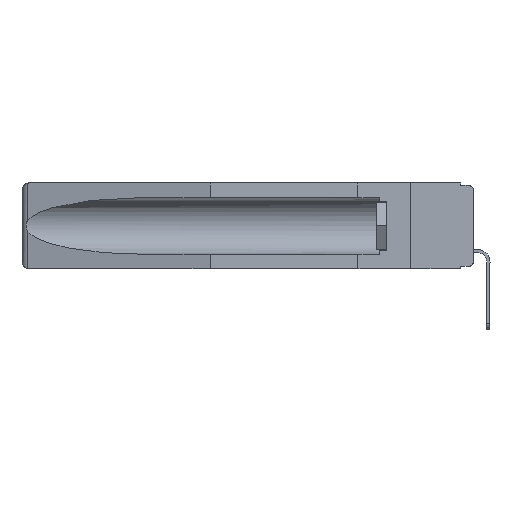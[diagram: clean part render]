
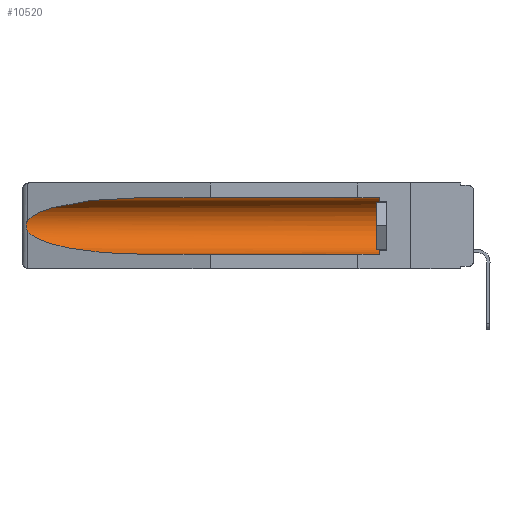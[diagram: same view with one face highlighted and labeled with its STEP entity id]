
A CAD part, left-side view. The second image highlights one B-rep face of the part: STEP entity #10520.
In plain terms, the highlighted cylindrical face has radius 2.857 mm (diameter 5.715 mm), a partial arc.
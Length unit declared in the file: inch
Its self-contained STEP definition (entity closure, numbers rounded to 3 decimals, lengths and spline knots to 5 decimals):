
#269 = VERTEX_POINT ( 'NONE', #14344 ) ;
#303 = DIRECTION ( 'NONE',  ( 0., 1., 0. ) ) ;
#357 = CYLINDRICAL_SURFACE ( 'NONE', #995, 0.1125 ) ;
#407 = CARTESIAN_POINT ( 'NONE',  ( 0.2675, 1.53308, -0.16763 ) ) ;
#995 = AXIS2_PLACEMENT_3D ( 'NONE', #14981, #9896, #12341 ) ;
#1066 = VECTOR ( 'NONE', #303, 39.37008 ) ;
#1364 = VERTEX_POINT ( 'NONE', #14664 ) ;
#1693 = EDGE_CURVE ( 'NONE', #8543, #269, #13814, .T. ) ;
#2449 = EDGE_CURVE ( 'NONE', #1364, #11812, #15150, .T. ) ;
#2573 = CARTESIAN_POINT ( 'NONE',  ( 0.155, 0.126, -0.1715 ) ) ;
#2664 = VERTEX_POINT ( 'NONE', #16634 ) ;
#2961 = CARTESIAN_POINT ( 'NONE',  ( 0.26537, 1.52718, -0.19328 ) ) ;
#3813 = CARTESIAN_POINT ( 'NONE',  ( 0.25451, 1.48313, -0.24835 ) ) ;
#4044 = ORIENTED_EDGE ( 'NONE', *, *, #7156, .T. ) ;
#4131 = ORIENTED_EDGE ( 'NONE', *, *, #1693, .T. ) ;
#4334 = CARTESIAN_POINT ( 'NONE',  ( 0.155, -0.30754, -0.284 ) ) ;
#4537 = CARTESIAN_POINT ( 'NONE',  ( 0.26597, 1.5296, -0.19026 ) ) ;
#4925 = CARTESIAN_POINT ( 'NONE',  ( 0.155, 1.07973, -0.059 ) ) ;
#6120 = CARTESIAN_POINT ( 'NONE',  ( 0.155, -0.30754, -0.059 ) ) ;
#6208 = ORIENTED_EDGE ( 'NONE', *, *, #2449, .T. ) ;
#6341 = CARTESIAN_POINT ( 'NONE',  ( 0.25451, 1.48313, -0.09465 ) ) ;
#6611 = DIRECTION ( 'NONE',  ( 0., -1., 0. ) ) ;
#7156 = EDGE_CURVE ( 'NONE', #2664, #10447, #7254, .T. ) ;
#7173 = CARTESIAN_POINT ( 'NONE',  ( 0.26597, 1.52961, -0.15275 ) ) ;
#7254 =( BOUNDED_CURVE ( )  B_SPLINE_CURVE ( 3, ( #10452, #3813, #14580, #13158 ),
 .UNSPECIFIED., .F., .F. ) 
 B_SPLINE_CURVE_WITH_KNOTS ( ( 4, 4 ),
 ( 0.1948, 1.5708 ),
 .UNSPECIFIED. ) 
 CURVE ( )  GEOMETRIC_REPRESENTATION_ITEM ( )  RATIONAL_B_SPLINE_CURVE ( ( 1., 0.848, 0.848, 1. ) ) 
 REPRESENTATION_ITEM ( '' )  );
#7483 = CARTESIAN_POINT ( 'NONE',  ( 0.26654, 1.53092, -0.15636 ) ) ;
#8113 = CARTESIAN_POINT ( 'NONE',  ( 0.155, 1.07973, -0.059 ) ) ;
#8366 = EDGE_CURVE ( 'NONE', #11812, #8543, #8810, .T. ) ;
#8543 = VERTEX_POINT ( 'NONE', #8113 ) ;
#8810 = LINE ( 'NONE', #6120, #15738 ) ;
#8953 = CARTESIAN_POINT ( 'NONE',  ( 0.21114, 1.30732, -0.059 ) ) ;
#9600 = CARTESIAN_POINT ( 'NONE',  ( 0.2673, 1.5327, -0.16383 ) ) ;
#9896 = DIRECTION ( 'NONE',  ( 0., 1., 0. ) ) ;
#9947 = DIRECTION ( 'NONE',  ( 0., 1., 0. ) ) ;
#10447 = VERTEX_POINT ( 'NONE', #10863 ) ;
#10452 = CARTESIAN_POINT ( 'NONE',  ( 0.26537, 1.52718, -0.19328 ) ) ;
#10520 = ADVANCED_FACE ( 'NONE', ( #16368 ), #357, .F. ) ;
#10704 = DIRECTION ( 'NONE',  ( 0., 0., 1. ) ) ;
#10769 = ORIENTED_EDGE ( 'NONE', *, *, #8366, .T. ) ;
#10863 = CARTESIAN_POINT ( 'NONE',  ( 0.155, 1.07973, -0.284 ) ) ;
#10994 = CARTESIAN_POINT ( 'NONE',  ( 0.2673, 1.53269, -0.17917 ) ) ;
#11036 = CARTESIAN_POINT ( 'NONE',  ( 0.155, 0.126, -0.059 ) ) ;
#11812 = VERTEX_POINT ( 'NONE', #11036 ) ;
#12341 = DIRECTION ( 'NONE',  ( 0., 0., 1. ) ) ;
#12583 = EDGE_CURVE ( 'NONE', #269, #2664, #13224, .T. ) ;
#12782 = ORIENTED_EDGE ( 'NONE', *, *, #12583, .T. ) ;
#13158 = CARTESIAN_POINT ( 'NONE',  ( 0.155, 1.07973, -0.284 ) ) ;
#13224 = B_SPLINE_CURVE_WITH_KNOTS ( 'NONE', 3,
 ( #13619, #7173, #7483, #9600, #407, #16152, #10994, #14943, #4537, #2961 ),
 .UNSPECIFIED., .F., .F.,
 ( 4, 2, 2, 2, 4 ),
 ( 0., 0.00029, 0.00058, 0.00087, 0.00117 ),
 .UNSPECIFIED. ) ;
#13619 = CARTESIAN_POINT ( 'NONE',  ( 0.26537, 1.52718, -0.14972 ) ) ;
#13814 =( BOUNDED_CURVE ( )  B_SPLINE_CURVE ( 3, ( #4925, #8953, #6341, #15592 ),
 .UNSPECIFIED., .F., .F. ) 
 B_SPLINE_CURVE_WITH_KNOTS ( ( 4, 4 ),
 ( 4.71239, 6.08839 ),
 .UNSPECIFIED. ) 
 CURVE ( )  GEOMETRIC_REPRESENTATION_ITEM ( )  RATIONAL_B_SPLINE_CURVE ( ( 1., 0.848, 0.848, 1. ) ) 
 REPRESENTATION_ITEM ( '' )  );
#13868 = LINE ( 'NONE', #4334, #1066 ) ;
#14301 = ORIENTED_EDGE ( 'NONE', *, *, #15737, .F. ) ;
#14344 = CARTESIAN_POINT ( 'NONE',  ( 0.26537, 1.52718, -0.14972 ) ) ;
#14580 = CARTESIAN_POINT ( 'NONE',  ( 0.21114, 1.30732, -0.284 ) ) ;
#14627 = EDGE_LOOP ( 'NONE', ( #4131, #12782, #4044, #14301, #6208, #10769 ) ) ;
#14664 = CARTESIAN_POINT ( 'NONE',  ( 0.155, 0.126, -0.284 ) ) ;
#14943 = CARTESIAN_POINT ( 'NONE',  ( 0.26655, 1.53094, -0.18657 ) ) ;
#14981 = CARTESIAN_POINT ( 'NONE',  ( 0.155, -0.30754, -0.1715 ) ) ;
#15150 = CIRCLE ( 'NONE', #17075, 0.1125 ) ;
#15592 = CARTESIAN_POINT ( 'NONE',  ( 0.26537, 1.52718, -0.14972 ) ) ;
#15737 = EDGE_CURVE ( 'NONE', #1364, #10447, #13868, .T. ) ;
#15738 = VECTOR ( 'NONE', #9947, 39.37008 ) ;
#16152 = CARTESIAN_POINT ( 'NONE',  ( 0.2675, 1.53308, -0.17534 ) ) ;
#16368 = FACE_OUTER_BOUND ( 'NONE', #14627, .T. ) ;
#16634 = CARTESIAN_POINT ( 'NONE',  ( 0.26537, 1.52718, -0.19328 ) ) ;
#17075 = AXIS2_PLACEMENT_3D ( 'NONE', #2573, #6611, #10704 ) ;
